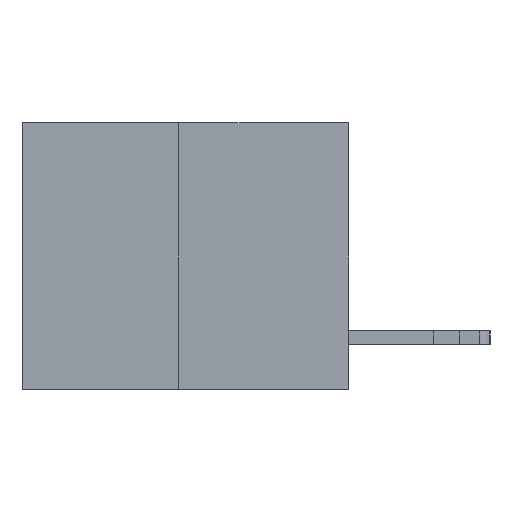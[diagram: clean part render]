
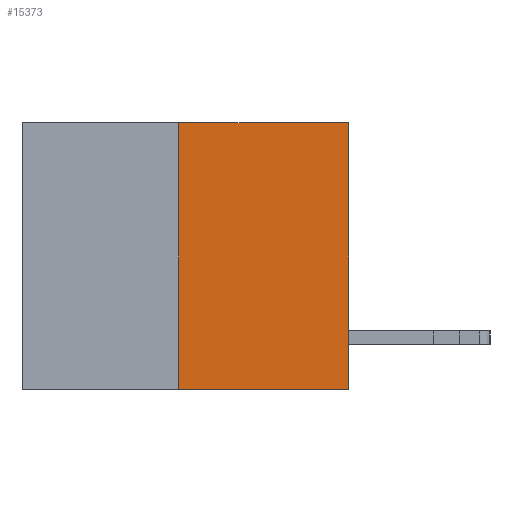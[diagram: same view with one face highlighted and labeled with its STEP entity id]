
A CAD part, left-side view. The second image highlights one B-rep face of the part: STEP entity #15373.
In plain terms, the highlighted planar face has unit normal (-1, 0, 0).
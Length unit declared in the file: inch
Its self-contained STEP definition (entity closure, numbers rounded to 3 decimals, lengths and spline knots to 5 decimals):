
#1020 = EDGE_CURVE ( 'NONE', #17965, #14371, #22701, .T. ) ;
#1604 = EDGE_CURVE ( 'NONE', #3871, #17965, #27019, .T. ) ;
#1910 = CARTESIAN_POINT ( 'NONE',  ( 0., 0.6, -0.49 ) ) ;
#3693 = DIRECTION ( 'NONE',  ( 0., 0., 1. ) ) ;
#3871 = VERTEX_POINT ( 'NONE', #24105 ) ;
#4929 = VECTOR ( 'NONE', #12684, 39.37008 ) ;
#5370 = EDGE_CURVE ( 'NONE', #20672, #14371, #26532, .T. ) ;
#6070 = CARTESIAN_POINT ( 'NONE',  ( 0., 0.6, 0. ) ) ;
#6570 = VECTOR ( 'NONE', #19345, 39.37008 ) ;
#6769 = CARTESIAN_POINT ( 'NONE',  ( 0., 0.312, 0. ) ) ;
#10802 = CARTESIAN_POINT ( 'NONE',  ( 0., 0.312, -0.49 ) ) ;
#12684 = DIRECTION ( 'NONE',  ( 0., -1., 0. ) ) ;
#13786 = VECTOR ( 'NONE', #19038, 39.37008 ) ;
#14182 = CARTESIAN_POINT ( 'NONE',  ( 0., 0., -0.49 ) ) ;
#14371 = VERTEX_POINT ( 'NONE', #24814 ) ;
#14415 = DIRECTION ( 'NONE',  ( 0., 0., -1. ) ) ;
#15373 = ADVANCED_FACE ( 'NONE', ( #19454 ), #23119, .F. ) ;
#17965 = VERTEX_POINT ( 'NONE', #6769 ) ;
#19038 = DIRECTION ( 'NONE',  ( 0., -1., 0. ) ) ;
#19345 = DIRECTION ( 'NONE',  ( 0., 0., 1. ) ) ;
#19454 = FACE_OUTER_BOUND ( 'NONE', #22395, .T. ) ;
#20433 = ORIENTED_EDGE ( 'NONE', *, *, #5370, .T. ) ;
#20672 = VERTEX_POINT ( 'NONE', #14182 ) ;
#20826 = LINE ( 'NONE', #1910, #13786 ) ;
#21206 = CARTESIAN_POINT ( 'NONE',  ( 0., 0.6, 0. ) ) ;
#21221 = AXIS2_PLACEMENT_3D ( 'NONE', #6070, #27236, #14415 ) ;
#22395 = EDGE_LOOP ( 'NONE', ( #26461, #27261, #20433, #25681 ) ) ;
#22701 = LINE ( 'NONE', #21206, #4929 ) ;
#23119 = PLANE ( 'NONE',  #21221 ) ;
#24105 = CARTESIAN_POINT ( 'NONE',  ( 0., 0.312, -0.49 ) ) ;
#24814 = CARTESIAN_POINT ( 'NONE',  ( 0., 0., 0. ) ) ;
#24838 = CARTESIAN_POINT ( 'NONE',  ( 0., 0., 0. ) ) ;
#25226 = VECTOR ( 'NONE', #3693, 39.37008 ) ;
#25681 = ORIENTED_EDGE ( 'NONE', *, *, #1020, .F. ) ;
#25703 = EDGE_CURVE ( 'NONE', #3871, #20672, #20826, .T. ) ;
#26461 = ORIENTED_EDGE ( 'NONE', *, *, #1604, .F. ) ;
#26532 = LINE ( 'NONE', #24838, #25226 ) ;
#27019 = LINE ( 'NONE', #10802, #6570 ) ;
#27236 = DIRECTION ( 'NONE',  ( 1., 0., 0. ) ) ;
#27261 = ORIENTED_EDGE ( 'NONE', *, *, #25703, .T. ) ;
